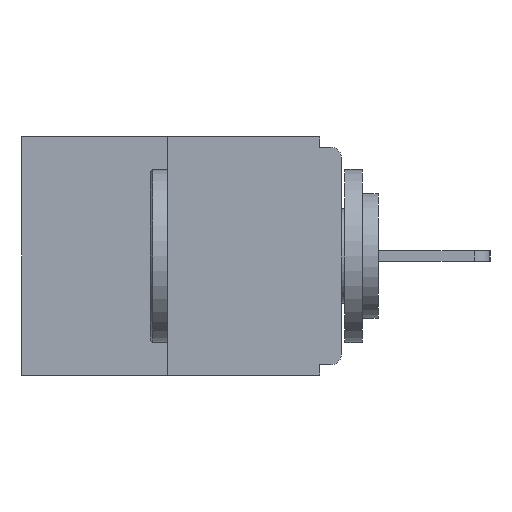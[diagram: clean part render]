
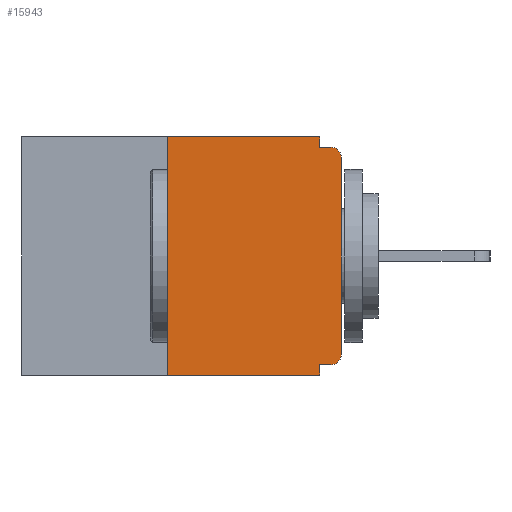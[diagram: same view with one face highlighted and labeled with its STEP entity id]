
A CAD part, left-side view. The second image highlights one B-rep face of the part: STEP entity #15943.
In plain terms, the highlighted planar face has unit normal (-1, 0, 0).
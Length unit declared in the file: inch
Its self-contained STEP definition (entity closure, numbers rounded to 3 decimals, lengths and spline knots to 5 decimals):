
#57 = LINE ( 'NONE', #16100, #14297 ) ;
#328 = CIRCLE ( 'NONE', #2198, 0.015 ) ;
#477 = EDGE_CURVE ( 'NONE', #5665, #2042, #10380, .T. ) ;
#590 = VERTEX_POINT ( 'NONE', #15056 ) ;
#670 = EDGE_CURVE ( 'NONE', #9208, #2042, #2059, .T. ) ;
#780 = LINE ( 'NONE', #10957, #13198 ) ;
#889 = EDGE_CURVE ( 'NONE', #5665, #12219, #4206, .T. ) ;
#923 = CARTESIAN_POINT ( 'NONE',  ( 0., 0.015, -0.313 ) ) ;
#1436 = VECTOR ( 'NONE', #6193, 39.37008 ) ;
#1697 = ORIENTED_EDGE ( 'NONE', *, *, #15229, .F. ) ;
#2042 = VERTEX_POINT ( 'NONE', #17668 ) ;
#2059 = LINE ( 'NONE', #13975, #8465 ) ;
#2066 = CIRCLE ( 'NONE', #13922, 0.015 ) ;
#2198 = AXIS2_PLACEMENT_3D ( 'NONE', #923, #12658, #15670 ) ;
#2547 = DIRECTION ( 'NONE',  ( 0., -1., 0. ) ) ;
#2644 = DIRECTION ( 'NONE',  ( 0., 0., 1. ) ) ;
#2921 = ORIENTED_EDGE ( 'NONE', *, *, #477, .T. ) ;
#3127 = ORIENTED_EDGE ( 'NONE', *, *, #15773, .F. ) ;
#3144 = ORIENTED_EDGE ( 'NONE', *, *, #6142, .F. ) ;
#3166 = VERTEX_POINT ( 'NONE', #12624 ) ;
#3625 = CARTESIAN_POINT ( 'NONE',  ( 0., 0.25, 0. ) ) ;
#3806 = DIRECTION ( 'NONE',  ( 0., 1., 0. ) ) ;
#4206 = LINE ( 'NONE', #13193, #11912 ) ;
#4897 = VERTEX_POINT ( 'NONE', #12388 ) ;
#4904 = ORIENTED_EDGE ( 'NONE', *, *, #10942, .T. ) ;
#5574 = DIRECTION ( 'NONE',  ( -1., 0., 0. ) ) ;
#5665 = VERTEX_POINT ( 'NONE', #17402 ) ;
#5867 = DIRECTION ( 'NONE',  ( 0., 0., -1. ) ) ;
#5925 = ORIENTED_EDGE ( 'NONE', *, *, #670, .F. ) ;
#6142 = EDGE_CURVE ( 'NONE', #3166, #9208, #18847, .T. ) ;
#6193 = DIRECTION ( 'NONE',  ( 0., -1., 0. ) ) ;
#6224 = ORIENTED_EDGE ( 'NONE', *, *, #17243, .T. ) ;
#6561 = DIRECTION ( 'NONE',  ( 0., 0., -1. ) ) ;
#7114 = DIRECTION ( 'NONE',  ( 0., 0., -1. ) ) ;
#7427 = ORIENTED_EDGE ( 'NONE', *, *, #8172, .T. ) ;
#7579 = CARTESIAN_POINT ( 'NONE',  ( 0., 0., -0.313 ) ) ;
#8172 = EDGE_CURVE ( 'NONE', #3166, #16414, #328, .T. ) ;
#8319 = CARTESIAN_POINT ( 'NONE',  ( 0., 0.46, 0. ) ) ;
#8324 = AXIS2_PLACEMENT_3D ( 'NONE', #8801, #14018, #5867 ) ;
#8420 = VECTOR ( 'NONE', #3806, 39.37008 ) ;
#8465 = VECTOR ( 'NONE', #6561, 39.37008 ) ;
#8629 = CARTESIAN_POINT ( 'NONE',  ( 0., 0.031, 0. ) ) ;
#8801 = CARTESIAN_POINT ( 'NONE',  ( 0., 0.46, 0. ) ) ;
#8880 = VERTEX_POINT ( 'NONE', #10841 ) ;
#9208 = VERTEX_POINT ( 'NONE', #14057 ) ;
#10380 = LINE ( 'NONE', #19070, #14587 ) ;
#10480 = DIRECTION ( 'NONE',  ( 0., -1., 0. ) ) ;
#10841 = CARTESIAN_POINT ( 'NONE',  ( 0., 0., -0.03 ) ) ;
#10894 = LINE ( 'NONE', #18222, #1436 ) ;
#10942 = EDGE_CURVE ( 'NONE', #16414, #8880, #780, .T. ) ;
#10957 = CARTESIAN_POINT ( 'NONE',  ( 0., 0., 0. ) ) ;
#11298 = ORIENTED_EDGE ( 'NONE', *, *, #889, .F. ) ;
#11912 = VECTOR ( 'NONE', #2644, 39.37008 ) ;
#12219 = VERTEX_POINT ( 'NONE', #3625 ) ;
#12388 = CARTESIAN_POINT ( 'NONE',  ( 0., 0.015, -0.015 ) ) ;
#12604 = DIRECTION ( 'NONE',  ( 0., 0., 1. ) ) ;
#12624 = CARTESIAN_POINT ( 'NONE',  ( 0., 0.015, -0.328 ) ) ;
#12658 = DIRECTION ( 'NONE',  ( -1., 0., 0. ) ) ;
#13193 = CARTESIAN_POINT ( 'NONE',  ( 0., 0.25, 0. ) ) ;
#13196 = FACE_OUTER_BOUND ( 'NONE', #16224, .T. ) ;
#13198 = VECTOR ( 'NONE', #12604, 39.37008 ) ;
#13922 = AXIS2_PLACEMENT_3D ( 'NONE', #17387, #5574, #14069 ) ;
#13975 = CARTESIAN_POINT ( 'NONE',  ( 0., 0.031, -0.343 ) ) ;
#14018 = DIRECTION ( 'NONE',  ( 1., 0., 0. ) ) ;
#14057 = CARTESIAN_POINT ( 'NONE',  ( 0., 0.031, -0.328 ) ) ;
#14069 = DIRECTION ( 'NONE',  ( 0., 0., -1. ) ) ;
#14297 = VECTOR ( 'NONE', #7114, 39.37008 ) ;
#14587 = VECTOR ( 'NONE', #10480, 39.37008 ) ;
#14753 = PLANE ( 'NONE',  #8324 ) ;
#14844 = ORIENTED_EDGE ( 'NONE', *, *, #19137, .F. ) ;
#15056 = CARTESIAN_POINT ( 'NONE',  ( 0., 0.031, -0.015 ) ) ;
#15229 = EDGE_CURVE ( 'NONE', #590, #4897, #10894, .T. ) ;
#15670 = DIRECTION ( 'NONE',  ( 0., 0., -1. ) ) ;
#15773 = EDGE_CURVE ( 'NONE', #12219, #16666, #17101, .T. ) ;
#15943 = ADVANCED_FACE ( 'NONE', ( #13196 ), #14753, .F. ) ;
#16100 = CARTESIAN_POINT ( 'NONE',  ( 0., 0.031, 0. ) ) ;
#16224 = EDGE_LOOP ( 'NONE', ( #3127, #11298, #2921, #5925, #3144, #7427, #4904, #6224, #1697, #14844 ) ) ;
#16414 = VERTEX_POINT ( 'NONE', #7579 ) ;
#16666 = VERTEX_POINT ( 'NONE', #8629 ) ;
#17101 = LINE ( 'NONE', #8319, #18617 ) ;
#17180 = CARTESIAN_POINT ( 'NONE',  ( 0., 0., -0.328 ) ) ;
#17243 = EDGE_CURVE ( 'NONE', #8880, #4897, #2066, .T. ) ;
#17387 = CARTESIAN_POINT ( 'NONE',  ( 0., 0.015, -0.03 ) ) ;
#17402 = CARTESIAN_POINT ( 'NONE',  ( 0., 0.25, -0.343 ) ) ;
#17668 = CARTESIAN_POINT ( 'NONE',  ( 0., 0.031, -0.343 ) ) ;
#18222 = CARTESIAN_POINT ( 'NONE',  ( 0., 0., -0.015 ) ) ;
#18617 = VECTOR ( 'NONE', #2547, 39.37008 ) ;
#18847 = LINE ( 'NONE', #17180, #8420 ) ;
#19070 = CARTESIAN_POINT ( 'NONE',  ( 0., 0.46, -0.343 ) ) ;
#19137 = EDGE_CURVE ( 'NONE', #16666, #590, #57, .T. ) ;
